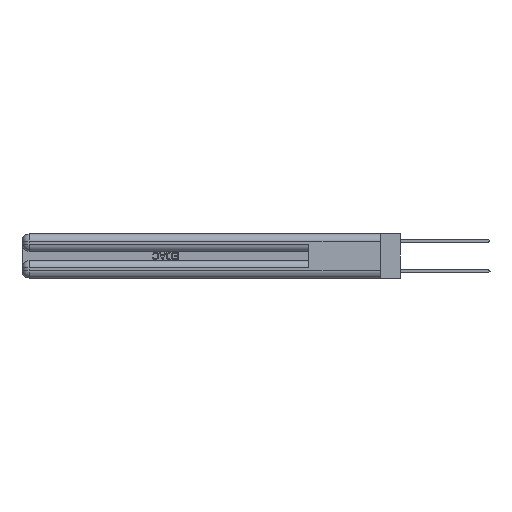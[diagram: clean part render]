
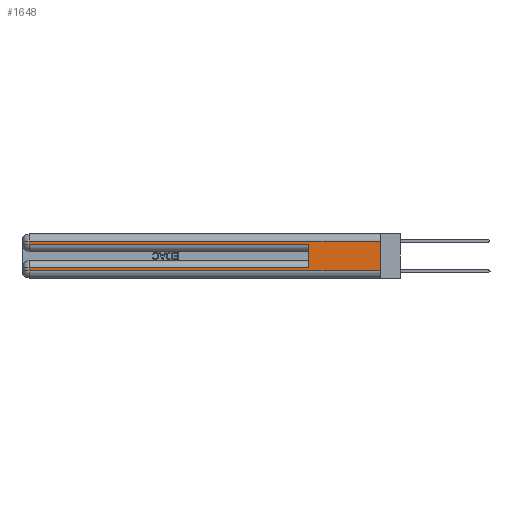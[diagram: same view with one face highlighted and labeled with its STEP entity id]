
A CAD part, left-side view. The second image highlights one B-rep face of the part: STEP entity #1648.
In plain terms, the highlighted planar face has unit normal (-1, 0, 0).
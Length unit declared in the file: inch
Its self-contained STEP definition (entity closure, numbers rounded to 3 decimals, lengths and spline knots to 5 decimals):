
#566 = CARTESIAN_POINT ( 'NONE',  ( 0., 2.94, 0.06 ) ) ;
#801 = VECTOR ( 'NONE', #16573, 39.37008 ) ;
#838 = VECTOR ( 'NONE', #3863, 39.37008 ) ;
#1023 = CARTESIAN_POINT ( 'NONE',  ( 0., 2.94, 0.37 ) ) ;
#1317 = CARTESIAN_POINT ( 'NONE',  ( 0., 0.6, 0.145 ) ) ;
#1648 = ADVANCED_FACE ( 'NONE', ( #27576 ), #15354, .F. ) ;
#1792 = CARTESIAN_POINT ( 'NONE',  ( 0., 0., 0.085 ) ) ;
#1887 = CARTESIAN_POINT ( 'NONE',  ( 0., 0.6, 0.085 ) ) ;
#2191 = VERTEX_POINT ( 'NONE', #26654 ) ;
#2224 = CARTESIAN_POINT ( 'NONE',  ( 0., 0., 0.37 ) ) ;
#2860 = CARTESIAN_POINT ( 'NONE',  ( 0., 2.94, 0.285 ) ) ;
#3863 = DIRECTION ( 'NONE',  ( 0., 0., -1. ) ) ;
#6492 = EDGE_CURVE ( 'NONE', #27357, #2191, #13483, .T. ) ;
#8166 = DIRECTION ( 'NONE',  ( 0., -1., 0. ) ) ;
#8409 = CARTESIAN_POINT ( 'NONE',  ( 0., 2.94, 0.31 ) ) ;
#8851 = ORIENTED_EDGE ( 'NONE', *, *, #10057, .T. ) ;
#8997 = EDGE_CURVE ( 'NONE', #14167, #30425, #27720, .T. ) ;
#9214 = EDGE_CURVE ( 'NONE', #30425, #19971, #26960, .T. ) ;
#10057 = EDGE_CURVE ( 'NONE', #20694, #27357, #21704, .T. ) ;
#10152 = EDGE_CURVE ( 'NONE', #17982, #28426, #33415, .T. ) ;
#10677 = LINE ( 'NONE', #13531, #29088 ) ;
#10732 = DIRECTION ( 'NONE',  ( 0., 0., -1. ) ) ;
#11592 = AXIS2_PLACEMENT_3D ( 'NONE', #35177, #29521, #26512 ) ;
#11612 = EDGE_CURVE ( 'NONE', #17982, #20694, #14895, .T. ) ;
#12968 = ORIENTED_EDGE ( 'NONE', *, *, #25049, .T. ) ;
#13483 = LINE ( 'NONE', #25019, #26321 ) ;
#13531 = CARTESIAN_POINT ( 'NONE',  ( 0., 0., 0.06 ) ) ;
#14167 = VERTEX_POINT ( 'NONE', #1887 ) ;
#14503 = DIRECTION ( 'NONE',  ( 0., 1., 0. ) ) ;
#14895 = LINE ( 'NONE', #31877, #17167 ) ;
#15354 = PLANE ( 'NONE',  #11592 ) ;
#16025 = ORIENTED_EDGE ( 'NONE', *, *, #10152, .F. ) ;
#16573 = DIRECTION ( 'NONE',  ( 0., 1., 0. ) ) ;
#17167 = VECTOR ( 'NONE', #14503, 39.37008 ) ;
#17982 = VERTEX_POINT ( 'NONE', #23003 ) ;
#18725 = LINE ( 'NONE', #1317, #32690 ) ;
#19260 = CARTESIAN_POINT ( 'NONE',  ( 0., 2.94, 0.085 ) ) ;
#19971 = VERTEX_POINT ( 'NONE', #566 ) ;
#20694 = VERTEX_POINT ( 'NONE', #8409 ) ;
#21704 = LINE ( 'NONE', #30217, #34085 ) ;
#22345 = ORIENTED_EDGE ( 'NONE', *, *, #9214, .T. ) ;
#22630 = VECTOR ( 'NONE', #10732, 39.37008 ) ;
#23003 = CARTESIAN_POINT ( 'NONE',  ( 0., 0., 0.31 ) ) ;
#23410 = ORIENTED_EDGE ( 'NONE', *, *, #11612, .T. ) ;
#24293 = ORIENTED_EDGE ( 'NONE', *, *, #30850, .F. ) ;
#25019 = CARTESIAN_POINT ( 'NONE',  ( 0., 0., 0.285 ) ) ;
#25049 = EDGE_CURVE ( 'NONE', #19971, #28426, #10677, .T. ) ;
#25070 = DIRECTION ( 'NONE',  ( 0., -1., 0. ) ) ;
#26321 = VECTOR ( 'NONE', #8166, 39.37008 ) ;
#26512 = DIRECTION ( 'NONE',  ( 0., 0., -1. ) ) ;
#26654 = CARTESIAN_POINT ( 'NONE',  ( 0., 0.6, 0.285 ) ) ;
#26770 = ORIENTED_EDGE ( 'NONE', *, *, #8997, .T. ) ;
#26886 = DIRECTION ( 'NONE',  ( 0., 0., 1. ) ) ;
#26960 = LINE ( 'NONE', #1023, #838 ) ;
#27357 = VERTEX_POINT ( 'NONE', #2860 ) ;
#27576 = FACE_OUTER_BOUND ( 'NONE', #30052, .T. ) ;
#27720 = LINE ( 'NONE', #1792, #801 ) ;
#28426 = VERTEX_POINT ( 'NONE', #34251 ) ;
#29088 = VECTOR ( 'NONE', #25070, 39.37008 ) ;
#29521 = DIRECTION ( 'NONE',  ( 1., 0., 0. ) ) ;
#30052 = EDGE_LOOP ( 'NONE', ( #16025, #23410, #8851, #35839, #24293, #26770, #22345, #12968 ) ) ;
#30217 = CARTESIAN_POINT ( 'NONE',  ( 0., 2.94, 0.37 ) ) ;
#30425 = VERTEX_POINT ( 'NONE', #19260 ) ;
#30779 = DIRECTION ( 'NONE',  ( 0., 0., -1. ) ) ;
#30850 = EDGE_CURVE ( 'NONE', #14167, #2191, #18725, .T. ) ;
#31877 = CARTESIAN_POINT ( 'NONE',  ( 0., 0., 0.31 ) ) ;
#32690 = VECTOR ( 'NONE', #26886, 39.37008 ) ;
#33415 = LINE ( 'NONE', #2224, #22630 ) ;
#34085 = VECTOR ( 'NONE', #30779, 39.37008 ) ;
#34251 = CARTESIAN_POINT ( 'NONE',  ( 0., 0., 0.06 ) ) ;
#35177 = CARTESIAN_POINT ( 'NONE',  ( 0., 0., 0.37 ) ) ;
#35839 = ORIENTED_EDGE ( 'NONE', *, *, #6492, .T. ) ;
